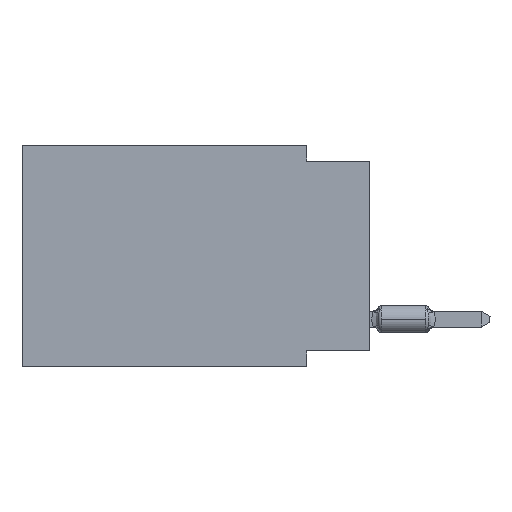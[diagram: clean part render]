
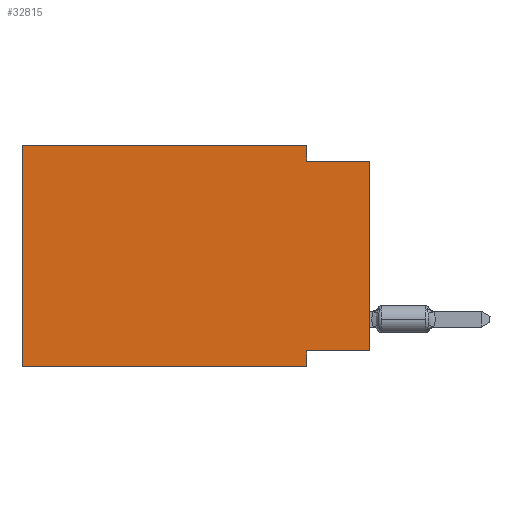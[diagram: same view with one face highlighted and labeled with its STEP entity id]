
A CAD part, left-side view. The second image highlights one B-rep face of the part: STEP entity #32815.
In plain terms, the highlighted planar face has unit normal (-1, 0, 0).
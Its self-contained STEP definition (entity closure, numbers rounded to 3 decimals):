
#972 = CARTESIAN_POINT ( 'NONE',  ( 0., 0., 0. ) ) ;
#1096 = ORIENTED_EDGE ( 'NONE', *, *, #12769, .F. ) ;
#2148 = CARTESIAN_POINT ( 'NONE',  ( 0., 0., -8.255 ) ) ;
#2330 = VERTEX_POINT ( 'NONE', #14813 ) ;
#2335 = EDGE_CURVE ( 'NONE', #2330, #18907, #14272, .T. ) ;
#2728 = CARTESIAN_POINT ( 'NONE',  ( 0., 2.54, 0. ) ) ;
#3287 = CARTESIAN_POINT ( 'NONE',  ( 0., 0., -0.635 ) ) ;
#3606 = EDGE_CURVE ( 'NONE', #27475, #35106, #31990, .T. ) ;
#3612 = PLANE ( 'NONE',  #34346 ) ;
#5563 = VECTOR ( 'NONE', #22711, 1000. ) ;
#6333 = FACE_OUTER_BOUND ( 'NONE', #30309, .T. ) ;
#6374 = DIRECTION ( 'NONE',  ( 0., -1., 0. ) ) ;
#6612 = DIRECTION ( 'NONE',  ( 0., 0., 1. ) ) ;
#7216 = CARTESIAN_POINT ( 'NONE',  ( 0., 2.54, -8.255 ) ) ;
#7312 = ORIENTED_EDGE ( 'NONE', *, *, #24332, .F. ) ;
#7372 = VECTOR ( 'NONE', #14778, 1000. ) ;
#8367 = LINE ( 'NONE', #33126, #30794 ) ;
#8979 = VERTEX_POINT ( 'NONE', #27379 ) ;
#9612 = CARTESIAN_POINT ( 'NONE',  ( 0., 13.97, -8.89 ) ) ;
#9628 = DIRECTION ( 'NONE',  ( 1., 0., 0. ) ) ;
#9689 = LINE ( 'NONE', #20056, #7372 ) ;
#9958 = DIRECTION ( 'NONE',  ( 0., 0., -1. ) ) ;
#10167 = DIRECTION ( 'NONE',  ( 0., 0., -1. ) ) ;
#11290 = VECTOR ( 'NONE', #6612, 1000. ) ;
#11867 = ORIENTED_EDGE ( 'NONE', *, *, #19038, .T. ) ;
#12328 = VERTEX_POINT ( 'NONE', #33531 ) ;
#12769 = EDGE_CURVE ( 'NONE', #12328, #8979, #8367, .T. ) ;
#12917 = ORIENTED_EDGE ( 'NONE', *, *, #3606, .F. ) ;
#13094 = ORIENTED_EDGE ( 'NONE', *, *, #21987, .F. ) ;
#14272 = LINE ( 'NONE', #972, #11290 ) ;
#14778 = DIRECTION ( 'NONE',  ( 0., -1., 0. ) ) ;
#14813 = CARTESIAN_POINT ( 'NONE',  ( 0., 0., -8.255 ) ) ;
#15424 = ORIENTED_EDGE ( 'NONE', *, *, #23261, .F. ) ;
#15578 = CARTESIAN_POINT ( 'NONE',  ( 0., 2.54, 0. ) ) ;
#17224 = LINE ( 'NONE', #35994, #5563 ) ;
#17608 = LINE ( 'NONE', #9612, #32913 ) ;
#18907 = VERTEX_POINT ( 'NONE', #33122 ) ;
#19038 = EDGE_CURVE ( 'NONE', #12328, #23165, #17608, .T. ) ;
#19981 = ORIENTED_EDGE ( 'NONE', *, *, #27290, .F. ) ;
#20056 = CARTESIAN_POINT ( 'NONE',  ( 0., 13.97, 0. ) ) ;
#20688 = ORIENTED_EDGE ( 'NONE', *, *, #2335, .T. ) ;
#21630 = DIRECTION ( 'NONE',  ( 0., 1., 0. ) ) ;
#21987 = EDGE_CURVE ( 'NONE', #2330, #34527, #27095, .T. ) ;
#22378 = VECTOR ( 'NONE', #9958, 1000. ) ;
#22711 = DIRECTION ( 'NONE',  ( 0., 0., -1. ) ) ;
#23165 = VERTEX_POINT ( 'NONE', #24024 ) ;
#23261 = EDGE_CURVE ( 'NONE', #34527, #23165, #17224, .T. ) ;
#24024 = CARTESIAN_POINT ( 'NONE',  ( 0., 2.54, -8.89 ) ) ;
#24332 = EDGE_CURVE ( 'NONE', #35106, #18907, #25691, .T. ) ;
#24571 = DIRECTION ( 'NONE',  ( 0., 0., 1. ) ) ;
#25455 = DIRECTION ( 'NONE',  ( 0., -1., 0. ) ) ;
#25691 = LINE ( 'NONE', #3287, #31312 ) ;
#27095 = LINE ( 'NONE', #2148, #33984 ) ;
#27290 = EDGE_CURVE ( 'NONE', #8979, #27475, #9689, .T. ) ;
#27379 = CARTESIAN_POINT ( 'NONE',  ( 0., 13.97, 0. ) ) ;
#27475 = VERTEX_POINT ( 'NONE', #2728 ) ;
#30309 = EDGE_LOOP ( 'NONE', ( #20688, #7312, #12917, #19981, #1096, #11867, #15424, #13094 ) ) ;
#30794 = VECTOR ( 'NONE', #24571, 1000. ) ;
#31312 = VECTOR ( 'NONE', #6374, 1000. ) ;
#31990 = LINE ( 'NONE', #15578, #22378 ) ;
#32815 = ADVANCED_FACE ( 'NONE', ( #6333 ), #3612, .F. ) ;
#32913 = VECTOR ( 'NONE', #25455, 1000. ) ;
#33122 = CARTESIAN_POINT ( 'NONE',  ( 0., 0., -0.635 ) ) ;
#33126 = CARTESIAN_POINT ( 'NONE',  ( 0., 13.97, 0. ) ) ;
#33531 = CARTESIAN_POINT ( 'NONE',  ( 0., 13.97, -8.89 ) ) ;
#33733 = CARTESIAN_POINT ( 'NONE',  ( 0., 2.54, -0.635 ) ) ;
#33984 = VECTOR ( 'NONE', #21630, 1000. ) ;
#34346 = AXIS2_PLACEMENT_3D ( 'NONE', #35270, #9628, #10167 ) ;
#34527 = VERTEX_POINT ( 'NONE', #7216 ) ;
#35106 = VERTEX_POINT ( 'NONE', #33733 ) ;
#35270 = CARTESIAN_POINT ( 'NONE',  ( 0., 13.97, 0. ) ) ;
#35994 = CARTESIAN_POINT ( 'NONE',  ( 0., 2.54, -8.89 ) ) ;
